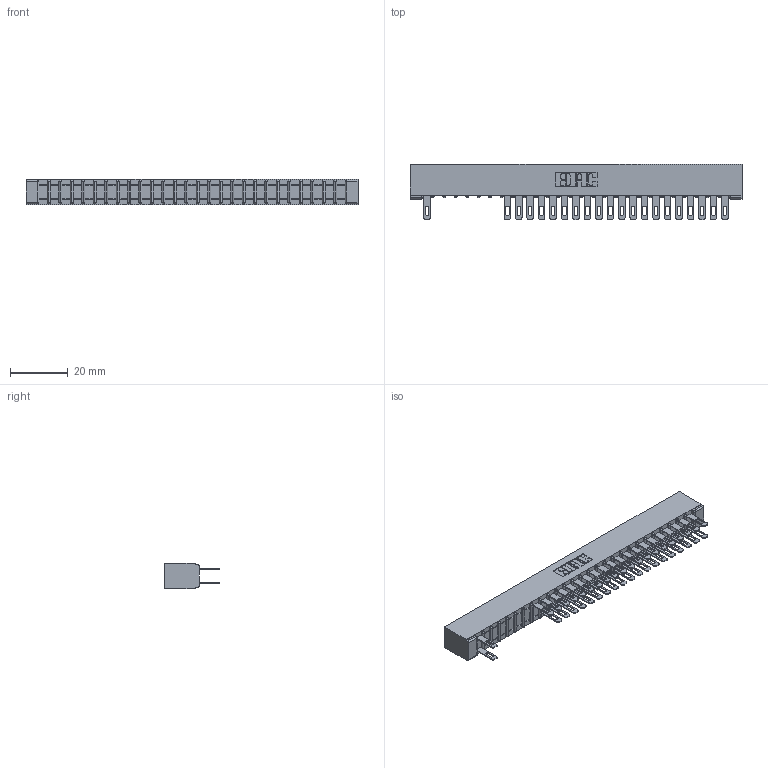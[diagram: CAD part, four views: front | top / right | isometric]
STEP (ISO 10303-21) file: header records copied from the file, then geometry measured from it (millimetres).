
FILE_DESCRIPTION (( 'STEP AP203' ), '1' );
FILE_NAME ('307-054-500-201.STEP', '2018-08-06T05:42:01', ( '' ), ( '' ), 'SwSTEP 2.0', 'SolidWorks 2016', '' );
FILE_SCHEMA (( 'CONFIG_CONTROL_DESIGN' ));
Length unit declared in the file: inch
Products named in the file (3): 307-290-001_500; 307-054-500-201; 307 Part_No Mounting Lugs
Assembly tree (42 placements, depth 2):
  307-054-500-201
    307 Part_No Mounting Lugs
    307-290-001_500  x41
Bounding box: 114.86 x 19.18 x 8.71 mm (x, y, z)
Volume: 7694.7 mm3; surface area: 13979.9 mm2
Topology: 42 solids, 42 shells, 2154 faces, 6045 edges, 3898 vertices
Faces by surface type: plane 1374, cylinder 724, sphere 56
Entity records: 25140 total; most frequent: CARTESIAN_POINT 4166, ORIENTED_EDGE 4138, DIRECTION 4075, EDGE_CURVE 2069, VECTOR 1581, LINE 1581, VERTEX_POINT 1338, AXIS2_PLACEMENT_3D 1247
